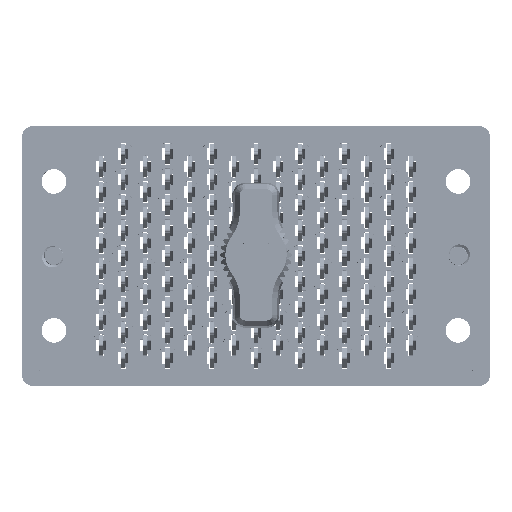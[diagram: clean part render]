
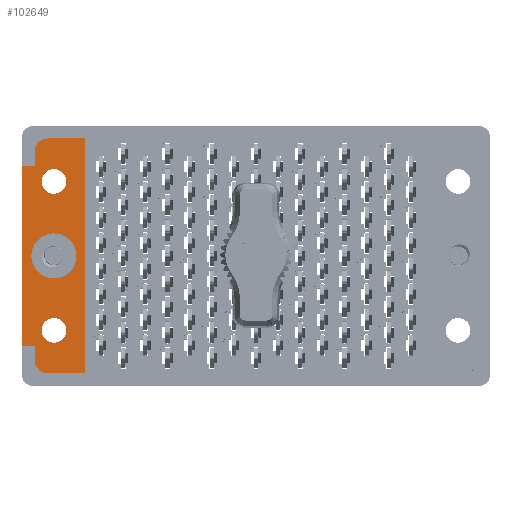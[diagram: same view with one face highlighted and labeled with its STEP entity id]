
A CAD part, top view. The second image highlights one B-rep face of the part: STEP entity #102649.
In plain terms, the highlighted planar face has unit normal (0, 0, 1).
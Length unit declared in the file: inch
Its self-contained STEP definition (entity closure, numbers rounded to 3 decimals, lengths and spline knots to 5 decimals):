
#366 = AXIS2_PLACEMENT_3D ( 'NONE', #25738, #8063, #7276 ) ;
#2274 = CIRCLE ( 'NONE', #366, 0.0725 ) ;
#3026 = VECTOR ( 'NONE', #23302, 39.37008 ) ;
#4818 = DIRECTION ( 'NONE',  ( -1., 0., 0. ) ) ;
#5773 = AXIS2_PLACEMENT_3D ( 'NONE', #39122, #12009, #75047 ) ;
#5942 = EDGE_CURVE ( 'NONE', #116147, #16368, #38076, .T. ) ;
#6301 = DIRECTION ( 'NONE',  ( 0., -1., 0. ) ) ;
#7276 = DIRECTION ( 'NONE',  ( 1., 0., 0. ) ) ;
#7817 = ORIENTED_EDGE ( 'NONE', *, *, #107531, .F. ) ;
#8063 = DIRECTION ( 'NONE',  ( 0., 0., 1. ) ) ;
#8523 = CARTESIAN_POINT ( 'NONE',  ( -1.3, 0.615, -0.117 ) ) ;
#9281 = CARTESIAN_POINT ( 'NONE',  ( -1.1875, 0., -0.117 ) ) ;
#9343 = CARTESIAN_POINT ( 'NONE',  ( -1.1875, 0.4375, -0.117 ) ) ;
#9423 = CARTESIAN_POINT ( 'NONE',  ( -1.005, -0.69, -0.117 ) ) ;
#9700 = LINE ( 'NONE', #25405, #73108 ) ;
#9737 = DIRECTION ( 'NONE',  ( 1., 0., 0. ) ) ;
#12009 = DIRECTION ( 'NONE',  ( 0., 0., 1. ) ) ;
#12892 = VERTEX_POINT ( 'NONE', #74567 ) ;
#13364 = CARTESIAN_POINT ( 'NONE',  ( -1.225, -0.69, -0.117 ) ) ;
#13879 = ORIENTED_EDGE ( 'NONE', *, *, #23331, .T. ) ;
#16149 = DIRECTION ( 'NONE',  ( 1., 0., 0. ) ) ;
#16368 = VERTEX_POINT ( 'NONE', #96798 ) ;
#16449 = DIRECTION ( 'NONE',  ( 0., 0., 1. ) ) ;
#17792 = EDGE_CURVE ( 'NONE', #16368, #49664, #99046, .T. ) ;
#18696 = CARTESIAN_POINT ( 'NONE',  ( -1.005, 0.69, -0.117 ) ) ;
#19504 = CIRCLE ( 'NONE', #69359, 0.075 ) ;
#19681 = CARTESIAN_POINT ( 'NONE',  ( 0., 0.69, -0.117 ) ) ;
#19900 = EDGE_CURVE ( 'NONE', #116147, #12892, #70481, .T. ) ;
#22152 = ORIENTED_EDGE ( 'NONE', *, *, #86966, .F. ) ;
#22225 = DIRECTION ( 'NONE',  ( -1., 0., 0. ) ) ;
#22658 = CIRCLE ( 'NONE', #114926, 0.0725 ) ;
#23302 = DIRECTION ( 'NONE',  ( -1., 0., 0. ) ) ;
#23331 = EDGE_CURVE ( 'NONE', #77885, #57877, #52708, .T. ) ;
#24826 = ORIENTED_EDGE ( 'NONE', *, *, #43438, .F. ) ;
#25405 = CARTESIAN_POINT ( 'NONE',  ( -1.3, 0., -0.117 ) ) ;
#25720 = CIRCLE ( 'NONE', #91692, 0.1325 ) ;
#25738 = CARTESIAN_POINT ( 'NONE',  ( -1.1875, -0.4375, -0.117 ) ) ;
#27403 = DIRECTION ( 'NONE',  ( 0., 0., 1. ) ) ;
#27410 = DIRECTION ( 'NONE',  ( 0., 0., 1. ) ) ;
#28693 = VECTOR ( 'NONE', #4818, 39.37008 ) ;
#30541 = VERTEX_POINT ( 'NONE', #44818 ) ;
#30928 = VECTOR ( 'NONE', #116215, 39.37008 ) ;
#32432 = EDGE_LOOP ( 'NONE', ( #56583, #90236 ) ) ;
#34242 = EDGE_CURVE ( 'NONE', #64777, #49664, #100276, .T. ) ;
#34844 = DIRECTION ( 'NONE',  ( 0., -1., 0. ) ) ;
#36044 = ORIENTED_EDGE ( 'NONE', *, *, #19900, .F. ) ;
#36174 = LINE ( 'NONE', #37484, #112287 ) ;
#36369 = DIRECTION ( 'NONE',  ( 1., 0., 0. ) ) ;
#36742 = AXIS2_PLACEMENT_3D ( 'NONE', #101063, #27403, #73520 ) ;
#37139 = CARTESIAN_POINT ( 'NONE',  ( -1.115, 0.4375, -0.117 ) ) ;
#37484 = CARTESIAN_POINT ( 'NONE',  ( -1.375, 0.7625, -0.117 ) ) ;
#38076 = LINE ( 'NONE', #60218, #84628 ) ;
#38117 = DIRECTION ( 'NONE',  ( 1., 0., 0. ) ) ;
#39122 = CARTESIAN_POINT ( 'NONE',  ( -1.1875, -0.4375, -0.117 ) ) ;
#39711 = CIRCLE ( 'NONE', #5773, 0.0725 ) ;
#41848 = FACE_BOUND ( 'NONE', #59000, .T. ) ;
#42371 = DIRECTION ( 'NONE',  ( 1., 0., 0. ) ) ;
#43255 = ORIENTED_EDGE ( 'NONE', *, *, #34242, .F. ) ;
#43438 = EDGE_CURVE ( 'NONE', #111659, #67483, #79635, .T. ) ;
#44012 = DIRECTION ( 'NONE',  ( 0., 0., 1. ) ) ;
#44102 = CARTESIAN_POINT ( 'NONE',  ( -1.005, 0.7625, -0.117 ) ) ;
#44511 = CIRCLE ( 'NONE', #109664, 0.0725 ) ;
#44818 = CARTESIAN_POINT ( 'NONE',  ( -1.26, 0.4375, -0.117 ) ) ;
#46305 = VECTOR ( 'NONE', #22225, 39.37008 ) ;
#46419 = EDGE_CURVE ( 'NONE', #94102, #30541, #22658, .T. ) ;
#49664 = VERTEX_POINT ( 'NONE', #13364 ) ;
#50568 = CARTESIAN_POINT ( 'NONE',  ( -1.26, -0.4375, -0.117 ) ) ;
#51029 = EDGE_CURVE ( 'NONE', #64777, #106090, #76113, .T. ) ;
#52708 = LINE ( 'NONE', #95354, #28693 ) ;
#53201 = FACE_BOUND ( 'NONE', #59439, .T. ) ;
#54179 = VECTOR ( 'NONE', #92950, 39.37008 ) ;
#56583 = ORIENTED_EDGE ( 'NONE', *, *, #86367, .F. ) ;
#56847 = DIRECTION ( 'NONE',  ( 0., 0., 1. ) ) ;
#57877 = VERTEX_POINT ( 'NONE', #81629 ) ;
#59000 = EDGE_LOOP ( 'NONE', ( #7817, #24826 ) ) ;
#59439 = EDGE_LOOP ( 'NONE', ( #71711, #22152 ) ) ;
#59522 = CARTESIAN_POINT ( 'NONE',  ( -1.3, -0.5285, -0.117 ) ) ;
#60218 = CARTESIAN_POINT ( 'NONE',  ( -1.3, 0., -0.117 ) ) ;
#61690 = ORIENTED_EDGE ( 'NONE', *, *, #95665, .T. ) ;
#62274 = EDGE_CURVE ( 'NONE', #57877, #12892, #36174, .T. ) ;
#64493 = ORIENTED_EDGE ( 'NONE', *, *, #51029, .T. ) ;
#64777 = VERTEX_POINT ( 'NONE', #9423 ) ;
#65124 = DIRECTION ( 'NONE',  ( 1., 0., 0. ) ) ;
#65597 = VERTEX_POINT ( 'NONE', #8523 ) ;
#65897 = ORIENTED_EDGE ( 'NONE', *, *, #84263, .T. ) ;
#67483 = VERTEX_POINT ( 'NONE', #111775 ) ;
#69021 = CARTESIAN_POINT ( 'NONE',  ( 0., -0.69, -0.117 ) ) ;
#69359 = AXIS2_PLACEMENT_3D ( 'NONE', #112787, #44012, #38117 ) ;
#70481 = LINE ( 'NONE', #84901, #46305 ) ;
#71711 = ORIENTED_EDGE ( 'NONE', *, *, #99874, .F. ) ;
#73108 = VECTOR ( 'NONE', #34844, 39.37008 ) ;
#73118 = CARTESIAN_POINT ( 'NONE',  ( -1.32, 0., -0.117 ) ) ;
#73520 = DIRECTION ( 'NONE',  ( 1., 0., 0. ) ) ;
#74567 = CARTESIAN_POINT ( 'NONE',  ( -1.375, -0.5285, -0.117 ) ) ;
#75047 = DIRECTION ( 'NONE',  ( 1., 0., 0. ) ) ;
#76113 = LINE ( 'NONE', #44102, #30928 ) ;
#77193 = FACE_BOUND ( 'NONE', #32432, .T. ) ;
#77885 = VERTEX_POINT ( 'NONE', #90780 ) ;
#78172 = LINE ( 'NONE', #19681, #54179 ) ;
#79635 = CIRCLE ( 'NONE', #86893, 0.1325 ) ;
#81629 = CARTESIAN_POINT ( 'NONE',  ( -1.375, 0.5285, -0.117 ) ) ;
#81664 = EDGE_CURVE ( 'NONE', #113428, #65597, #19504, .T. ) ;
#84263 = EDGE_CURVE ( 'NONE', #106090, #113428, #78172, .T. ) ;
#84628 = VECTOR ( 'NONE', #6301, 39.37008 ) ;
#84901 = CARTESIAN_POINT ( 'NONE',  ( 0., -0.5285, -0.117 ) ) ;
#86367 = EDGE_CURVE ( 'NONE', #30541, #94102, #44511, .T. ) ;
#86893 = AXIS2_PLACEMENT_3D ( 'NONE', #87857, #97669, #16149 ) ;
#86966 = EDGE_CURVE ( 'NONE', #114166, #87740, #2274, .T. ) ;
#87740 = VERTEX_POINT ( 'NONE', #50568 ) ;
#87857 = CARTESIAN_POINT ( 'NONE',  ( -1.1875, 0., -0.117 ) ) ;
#87939 = ORIENTED_EDGE ( 'NONE', *, *, #62274, .T. ) ;
#89107 = ORIENTED_EDGE ( 'NONE', *, *, #5942, .T. ) ;
#90236 = ORIENTED_EDGE ( 'NONE', *, *, #46419, .F. ) ;
#90763 = EDGE_LOOP ( 'NONE', ( #65897, #99346, #61690, #13879, #87939, #36044, #89107, #94502, #43255, #64493 ) ) ;
#90780 = CARTESIAN_POINT ( 'NONE',  ( -1.3, 0.5285, -0.117 ) ) ;
#91692 = AXIS2_PLACEMENT_3D ( 'NONE', #9281, #108479, #36369 ) ;
#92305 = DIRECTION ( 'NONE',  ( 0., -1., 0. ) ) ;
#92950 = DIRECTION ( 'NONE',  ( -1., 0., 0. ) ) ;
#94102 = VERTEX_POINT ( 'NONE', #37139 ) ;
#94502 = ORIENTED_EDGE ( 'NONE', *, *, #17792, .T. ) ;
#95079 = CARTESIAN_POINT ( 'NONE',  ( -1.115, -0.4375, -0.117 ) ) ;
#95354 = CARTESIAN_POINT ( 'NONE',  ( 0., 0.5285, -0.117 ) ) ;
#95665 = EDGE_CURVE ( 'NONE', #65597, #77885, #9700, .T. ) ;
#96798 = CARTESIAN_POINT ( 'NONE',  ( -1.3, -0.615, -0.117 ) ) ;
#97669 = DIRECTION ( 'NONE',  ( 0., 0., 1. ) ) ;
#98320 = FACE_OUTER_BOUND ( 'NONE', #90763, .T. ) ;
#99046 = CIRCLE ( 'NONE', #36742, 0.075 ) ;
#99346 = ORIENTED_EDGE ( 'NONE', *, *, #81664, .T. ) ;
#99874 = EDGE_CURVE ( 'NONE', #87740, #114166, #39711, .T. ) ;
#100276 = LINE ( 'NONE', #69021, #3026 ) ;
#101063 = CARTESIAN_POINT ( 'NONE',  ( -1.225, -0.615, -0.117 ) ) ;
#101366 = PLANE ( 'NONE',  #112323 ) ;
#102649 = ADVANCED_FACE ( 'NONE', ( #77193, #53201, #41848, #98320 ), #101366, .T. ) ;
#103549 = CARTESIAN_POINT ( 'NONE',  ( -1.225, 0.69, -0.117 ) ) ;
#105800 = CARTESIAN_POINT ( 'NONE',  ( -1.1875, 0.4375, -0.117 ) ) ;
#106090 = VERTEX_POINT ( 'NONE', #18696 ) ;
#107531 = EDGE_CURVE ( 'NONE', #67483, #111659, #25720, .T. ) ;
#108479 = DIRECTION ( 'NONE',  ( 0., 0., 1. ) ) ;
#109618 = CARTESIAN_POINT ( 'NONE',  ( -1.375, -0.7625, -0.117 ) ) ;
#109664 = AXIS2_PLACEMENT_3D ( 'NONE', #9343, #27410, #9737 ) ;
#111659 = VERTEX_POINT ( 'NONE', #73118 ) ;
#111775 = CARTESIAN_POINT ( 'NONE',  ( -1.055, 0., -0.117 ) ) ;
#112287 = VECTOR ( 'NONE', #92305, 39.37008 ) ;
#112323 = AXIS2_PLACEMENT_3D ( 'NONE', #109618, #56847, #65124 ) ;
#112787 = CARTESIAN_POINT ( 'NONE',  ( -1.225, 0.615, -0.117 ) ) ;
#113428 = VERTEX_POINT ( 'NONE', #103549 ) ;
#114166 = VERTEX_POINT ( 'NONE', #95079 ) ;
#114926 = AXIS2_PLACEMENT_3D ( 'NONE', #105800, #16449, #42371 ) ;
#116147 = VERTEX_POINT ( 'NONE', #59522 ) ;
#116215 = DIRECTION ( 'NONE',  ( 0., 1., 0. ) ) ;
